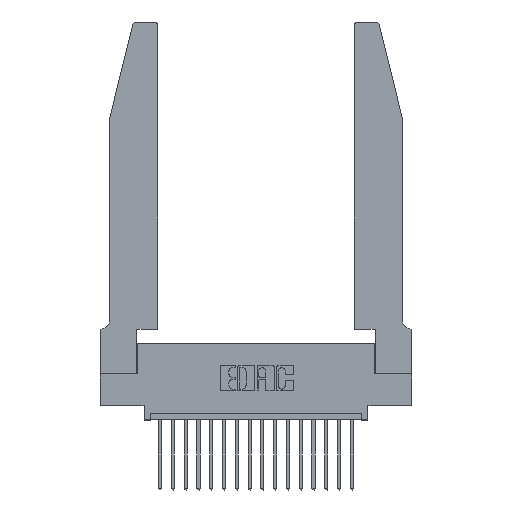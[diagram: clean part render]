
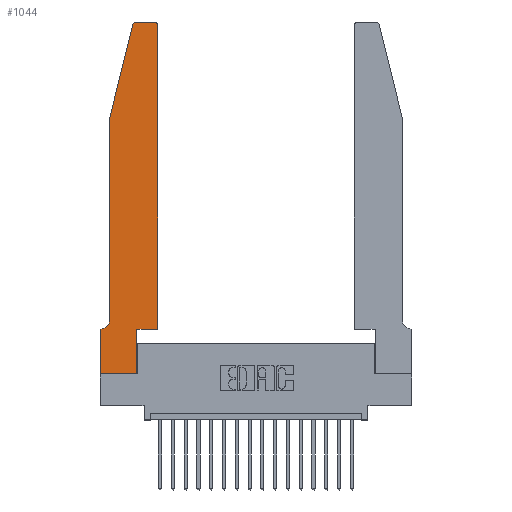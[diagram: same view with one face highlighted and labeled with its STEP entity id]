
A CAD part, top view. The second image highlights one B-rep face of the part: STEP entity #1044.
In plain terms, the highlighted planar face has unit normal (0, 0, 1).
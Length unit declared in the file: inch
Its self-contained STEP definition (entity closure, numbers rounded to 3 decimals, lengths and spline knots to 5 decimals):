
#175 = LINE ( 'NONE', #12951, #16940 ) ;
#491 = DIRECTION ( 'NONE',  ( 0., 0., -1. ) ) ;
#503 = CARTESIAN_POINT ( 'NONE',  ( 0.0755, 2., 0.37 ) ) ;
#1044 = ADVANCED_FACE ( 'NONE', ( #5816 ), #17061, .T. ) ;
#1641 = CARTESIAN_POINT ( 'NONE',  ( 0., 0., 0.37 ) ) ;
#1664 = DIRECTION ( 'NONE',  ( 1., 0., 0. ) ) ;
#1856 = EDGE_CURVE ( 'NONE', #20267, #15324, #14217, .T. ) ;
#2051 = CARTESIAN_POINT ( 'NONE',  ( 0.2865, 0.35, 0.37 ) ) ;
#2267 = AXIS2_PLACEMENT_3D ( 'NONE', #9435, #15639, #15776 ) ;
#2444 = CARTESIAN_POINT ( 'NONE',  ( 0.4505, 0.35, 0.37 ) ) ;
#2726 = ORIENTED_EDGE ( 'NONE', *, *, #17865, .T. ) ;
#2839 = VECTOR ( 'NONE', #9242, 39.37008 ) ;
#3092 = EDGE_CURVE ( 'NONE', #19853, #8911, #4757, .T. ) ;
#3137 = VECTOR ( 'NONE', #6515, 39.37008 ) ;
#3260 = LINE ( 'NONE', #8978, #12424 ) ;
#3318 = DIRECTION ( 'NONE',  ( 0., 0., 1. ) ) ;
#3777 = EDGE_CURVE ( 'NONE', #17607, #12769, #5230, .T. ) ;
#3794 = CIRCLE ( 'NONE', #2267, 0.03 ) ;
#3968 = ORIENTED_EDGE ( 'NONE', *, *, #3092, .T. ) ;
#3980 = CARTESIAN_POINT ( 'NONE',  ( 0.4505, 0.35, 0.37 ) ) ;
#4334 = VERTEX_POINT ( 'NONE', #19173 ) ;
#4418 = VECTOR ( 'NONE', #13854, 39.37008 ) ;
#4459 = ORIENTED_EDGE ( 'NONE', *, *, #14946, .T. ) ;
#4490 = AXIS2_PLACEMENT_3D ( 'NONE', #14436, #3318, #19157 ) ;
#4757 = CIRCLE ( 'NONE', #15393, 0.07 ) ;
#5230 = LINE ( 'NONE', #503, #12137 ) ;
#5291 = VECTOR ( 'NONE', #19716, 39.37008 ) ;
#5578 = CARTESIAN_POINT ( 'NONE',  ( 0.284, 2.75, 0.37 ) ) ;
#5609 = EDGE_CURVE ( 'NONE', #11924, #4334, #13543, .T. ) ;
#5816 = FACE_OUTER_BOUND ( 'NONE', #19667, .T. ) ;
#6090 = VERTEX_POINT ( 'NONE', #1641 ) ;
#6264 = DIRECTION ( 'NONE',  ( -1., 0., 0. ) ) ;
#6515 = DIRECTION ( 'NONE',  ( 0., -1., 0. ) ) ;
#6922 = DIRECTION ( 'NONE',  ( -1., 0., 0. ) ) ;
#6943 = EDGE_CURVE ( 'NONE', #12390, #13588, #12758, .T. ) ;
#7036 = EDGE_CURVE ( 'NONE', #15324, #17607, #13984, .T. ) ;
#7737 = CARTESIAN_POINT ( 'NONE',  ( 0.0755, 0.35, 0.37 ) ) ;
#8001 = CARTESIAN_POINT ( 'NONE',  ( 0., 0.35, 0.37 ) ) ;
#8506 = EDGE_CURVE ( 'NONE', #12769, #19853, #10336, .T. ) ;
#8911 = VERTEX_POINT ( 'NONE', #13711 ) ;
#8978 = CARTESIAN_POINT ( 'NONE',  ( 0.4505, 0.35, 0.37 ) ) ;
#9179 = ORIENTED_EDGE ( 'NONE', *, *, #3777, .T. ) ;
#9242 = DIRECTION ( 'NONE',  ( 0., 1., 0. ) ) ;
#9435 = CARTESIAN_POINT ( 'NONE',  ( 0.4205, 2.72, 0.37 ) ) ;
#9553 = DIRECTION ( 'NONE',  ( 0., 0., 1. ) ) ;
#10336 = LINE ( 'NONE', #14360, #3137 ) ;
#10347 = DIRECTION ( 'NONE',  ( 0., 1., 0. ) ) ;
#11017 = ORIENTED_EDGE ( 'NONE', *, *, #15299, .T. ) ;
#11218 = CARTESIAN_POINT ( 'NONE',  ( 0.4205, 2.75, 0.37 ) ) ;
#11924 = VERTEX_POINT ( 'NONE', #3980 ) ;
#12089 = LINE ( 'NONE', #7737, #4418 ) ;
#12137 = VECTOR ( 'NONE', #16937, 39.37008 ) ;
#12390 = VERTEX_POINT ( 'NONE', #20092 ) ;
#12424 = VECTOR ( 'NONE', #15440, 39.37008 ) ;
#12429 = EDGE_CURVE ( 'NONE', #13588, #11924, #3260, .T. ) ;
#12537 = CARTESIAN_POINT ( 'NONE',  ( 0.2605, 2.75, 0.37 ) ) ;
#12758 = LINE ( 'NONE', #2051, #2839 ) ;
#12769 = VERTEX_POINT ( 'NONE', #14455 ) ;
#12951 = CARTESIAN_POINT ( 'NONE',  ( 0., 0., 0.37 ) ) ;
#12992 = ORIENTED_EDGE ( 'NONE', *, *, #6943, .T. ) ;
#13474 = ORIENTED_EDGE ( 'NONE', *, *, #19757, .T. ) ;
#13543 = LINE ( 'NONE', #2444, #16992 ) ;
#13588 = VERTEX_POINT ( 'NONE', #18167 ) ;
#13711 = CARTESIAN_POINT ( 'NONE',  ( 0.0055, 0.35, 0.37 ) ) ;
#13854 = DIRECTION ( 'NONE',  ( -1., 0., 0. ) ) ;
#13984 = CIRCLE ( 'NONE', #4490, 0.03 ) ;
#14020 = CARTESIAN_POINT ( 'NONE',  ( 0., 0.35, 0.37 ) ) ;
#14217 = LINE ( 'NONE', #12537, #18646 ) ;
#14359 = ORIENTED_EDGE ( 'NONE', *, *, #8506, .T. ) ;
#14360 = CARTESIAN_POINT ( 'NONE',  ( 0.0755, 2., 0.37 ) ) ;
#14436 = CARTESIAN_POINT ( 'NONE',  ( 0.284, 2.72, 0.37 ) ) ;
#14455 = CARTESIAN_POINT ( 'NONE',  ( 0.0755, 2., 0.37 ) ) ;
#14946 = EDGE_CURVE ( 'NONE', #4334, #20267, #3794, .T. ) ;
#15299 = EDGE_CURVE ( 'NONE', #17435, #6090, #15656, .T. ) ;
#15324 = VERTEX_POINT ( 'NONE', #5578 ) ;
#15393 = AXIS2_PLACEMENT_3D ( 'NONE', #16349, #491, #6922 ) ;
#15440 = DIRECTION ( 'NONE',  ( 1., 0., 0. ) ) ;
#15639 = DIRECTION ( 'NONE',  ( 0., 0., 1. ) ) ;
#15656 = LINE ( 'NONE', #18128, #5291 ) ;
#15776 = DIRECTION ( 'NONE',  ( 1., 0., 0. ) ) ;
#16317 = AXIS2_PLACEMENT_3D ( 'NONE', #8001, #9553, #1664 ) ;
#16349 = CARTESIAN_POINT ( 'NONE',  ( 0.0055, 0.42, 0.37 ) ) ;
#16466 = CARTESIAN_POINT ( 'NONE',  ( 0.0755, 0.42, 0.37 ) ) ;
#16937 = DIRECTION ( 'NONE',  ( -0.239, -0.971, 0. ) ) ;
#16940 = VECTOR ( 'NONE', #19117, 39.37008 ) ;
#16992 = VECTOR ( 'NONE', #10347, 39.37008 ) ;
#17061 = PLANE ( 'NONE',  #16317 ) ;
#17435 = VERTEX_POINT ( 'NONE', #14020 ) ;
#17607 = VERTEX_POINT ( 'NONE', #18145 ) ;
#17865 = EDGE_CURVE ( 'NONE', #8911, #17435, #12089, .T. ) ;
#18128 = CARTESIAN_POINT ( 'NONE',  ( 0., 0., 0.37 ) ) ;
#18145 = CARTESIAN_POINT ( 'NONE',  ( 0.25487, 2.72718, 0.37 ) ) ;
#18167 = CARTESIAN_POINT ( 'NONE',  ( 0.2865, 0.35, 0.37 ) ) ;
#18577 = ORIENTED_EDGE ( 'NONE', *, *, #7036, .T. ) ;
#18640 = ORIENTED_EDGE ( 'NONE', *, *, #1856, .T. ) ;
#18646 = VECTOR ( 'NONE', #6264, 39.37008 ) ;
#19117 = DIRECTION ( 'NONE',  ( 1., 0., 0. ) ) ;
#19157 = DIRECTION ( 'NONE',  ( 1., 0., 0. ) ) ;
#19173 = CARTESIAN_POINT ( 'NONE',  ( 0.4505, 2.72, 0.37 ) ) ;
#19667 = EDGE_LOOP ( 'NONE', ( #18640, #18577, #9179, #14359, #3968, #2726, #11017, #13474, #12992, #20106, #19852, #4459 ) ) ;
#19716 = DIRECTION ( 'NONE',  ( 0., -1., 0. ) ) ;
#19757 = EDGE_CURVE ( 'NONE', #6090, #12390, #175, .T. ) ;
#19852 = ORIENTED_EDGE ( 'NONE', *, *, #5609, .T. ) ;
#19853 = VERTEX_POINT ( 'NONE', #16466 ) ;
#20092 = CARTESIAN_POINT ( 'NONE',  ( 0.2865, 0., 0.37 ) ) ;
#20106 = ORIENTED_EDGE ( 'NONE', *, *, #12429, .T. ) ;
#20267 = VERTEX_POINT ( 'NONE', #11218 ) ;
